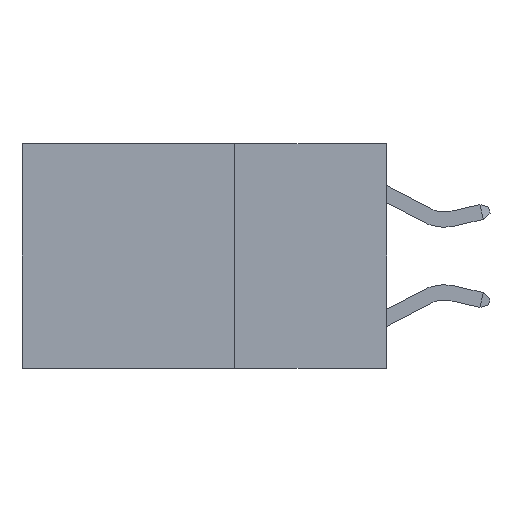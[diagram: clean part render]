
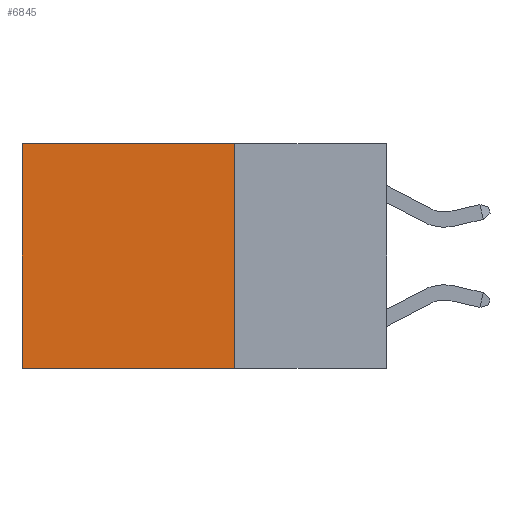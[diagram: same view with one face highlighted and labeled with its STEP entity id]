
A CAD part, left-side view. The second image highlights one B-rep face of the part: STEP entity #6845.
In plain terms, the highlighted planar face has unit normal (-1, 0, 0).
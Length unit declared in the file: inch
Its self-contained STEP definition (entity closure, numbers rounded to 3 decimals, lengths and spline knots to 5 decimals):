
#1083 = CARTESIAN_POINT ( 'NONE',  ( 0.2625, 0.25, 0. ) ) ;
#1528 = EDGE_CURVE ( 'NONE', #1830, #9131, #1781, .T. ) ;
#1561 = LINE ( 'NONE', #1774, #8571 ) ;
#1774 = CARTESIAN_POINT ( 'NONE',  ( 0.2625, 0.25, -0.37 ) ) ;
#1781 = LINE ( 'NONE', #1083, #9594 ) ;
#1830 = VERTEX_POINT ( 'NONE', #5771 ) ;
#1907 = CARTESIAN_POINT ( 'NONE',  ( 0.2625, 0.25, 0. ) ) ;
#2073 = CARTESIAN_POINT ( 'NONE',  ( 0.2625, 0.6, 0. ) ) ;
#2506 = DIRECTION ( 'NONE',  ( 0., 1., 0. ) ) ;
#2741 = PLANE ( 'NONE',  #4423 ) ;
#2833 = DIRECTION ( 'NONE',  ( 0., 0., -1. ) ) ;
#2839 = VECTOR ( 'NONE', #2833, 39.37008 ) ;
#3068 = ORIENTED_EDGE ( 'NONE', *, *, #1528, .T. ) ;
#3464 = FACE_OUTER_BOUND ( 'NONE', #9262, .T. ) ;
#4283 = DIRECTION ( 'NONE',  ( 0., 0., -1. ) ) ;
#4423 = AXIS2_PLACEMENT_3D ( 'NONE', #1907, #6463, #6430 ) ;
#5113 = CARTESIAN_POINT ( 'NONE',  ( 0.2625, 0.6, -0.37 ) ) ;
#5163 = CARTESIAN_POINT ( 'NONE',  ( 0.2625, 0.25, 0. ) ) ;
#5240 = CARTESIAN_POINT ( 'NONE',  ( 0.2625, 0.6, 0. ) ) ;
#5276 = EDGE_CURVE ( 'NONE', #9131, #9051, #7044, .T. ) ;
#5771 = CARTESIAN_POINT ( 'NONE',  ( 0.2625, 0.25, 0. ) ) ;
#6147 = LINE ( 'NONE', #5163, #2839 ) ;
#6430 = DIRECTION ( 'NONE',  ( 0., 0., -1. ) ) ;
#6463 = DIRECTION ( 'NONE',  ( 1., 0., 0. ) ) ;
#6733 = EDGE_CURVE ( 'NONE', #7173, #9051, #1561, .T. ) ;
#6845 = ADVANCED_FACE ( 'NONE', ( #3464 ), #2741, .F. ) ;
#6956 = EDGE_CURVE ( 'NONE', #1830, #7173, #6147, .T. ) ;
#7044 = LINE ( 'NONE', #2073, #8317 ) ;
#7173 = VERTEX_POINT ( 'NONE', #8304 ) ;
#7631 = ORIENTED_EDGE ( 'NONE', *, *, #6733, .F. ) ;
#7778 = ORIENTED_EDGE ( 'NONE', *, *, #5276, .T. ) ;
#8304 = CARTESIAN_POINT ( 'NONE',  ( 0.2625, 0.25, -0.37 ) ) ;
#8317 = VECTOR ( 'NONE', #4283, 39.37008 ) ;
#8571 = VECTOR ( 'NONE', #2506, 39.37008 ) ;
#9051 = VERTEX_POINT ( 'NONE', #5113 ) ;
#9131 = VERTEX_POINT ( 'NONE', #5240 ) ;
#9209 = DIRECTION ( 'NONE',  ( 0., 1., 0. ) ) ;
#9262 = EDGE_LOOP ( 'NONE', ( #7778, #7631, #9632, #3068 ) ) ;
#9594 = VECTOR ( 'NONE', #9209, 39.37008 ) ;
#9632 = ORIENTED_EDGE ( 'NONE', *, *, #6956, .F. ) ;
